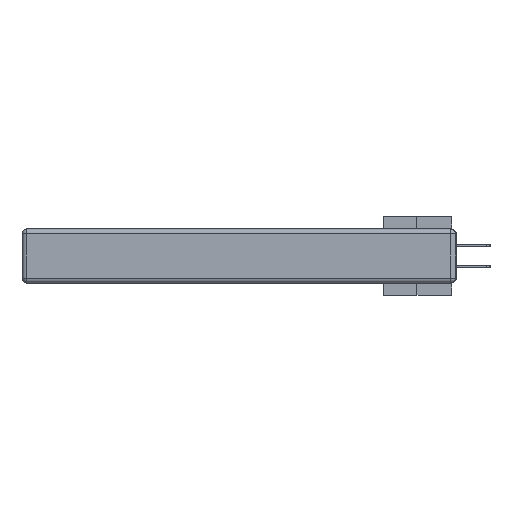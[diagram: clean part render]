
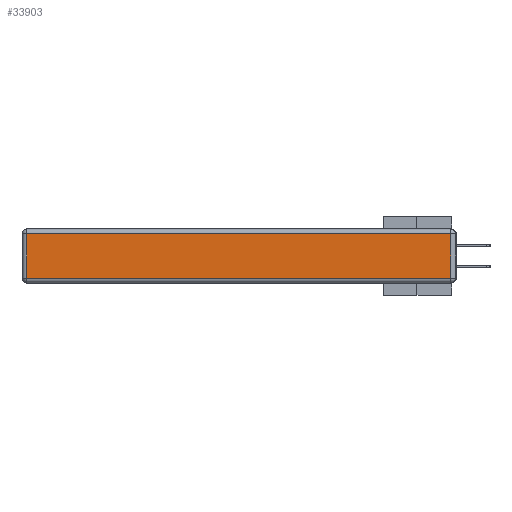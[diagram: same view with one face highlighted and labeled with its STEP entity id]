
A CAD part, left-side view. The second image highlights one B-rep face of the part: STEP entity #33903.
In plain terms, the highlighted planar face has unit normal (-1, 0, 0).
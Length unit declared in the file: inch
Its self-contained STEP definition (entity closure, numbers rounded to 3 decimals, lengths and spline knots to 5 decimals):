
#433 = VERTEX_POINT ( 'NONE', #36442 ) ;
#593 = DIRECTION ( 'NONE',  ( -1., 0., 0. ) ) ;
#1270 = ORIENTED_EDGE ( 'NONE', *, *, #34330, .T. ) ;
#1460 = DIRECTION ( 'NONE',  ( 0., 0., -1. ) ) ;
#1658 = VECTOR ( 'NONE', #24372, 39.37008 ) ;
#2230 = CARTESIAN_POINT ( 'NONE',  ( 0., 2.72, -0.313 ) ) ;
#3919 = ORIENTED_EDGE ( 'NONE', *, *, #25011, .T. ) ;
#5621 = EDGE_CURVE ( 'NONE', #29879, #16397, #23557, .T. ) ;
#6476 = CARTESIAN_POINT ( 'NONE',  ( 0., 2.72, -0.03 ) ) ;
#8736 = LINE ( 'NONE', #32435, #29764 ) ;
#9277 = VERTEX_POINT ( 'NONE', #2230 ) ;
#10388 = DIRECTION ( 'NONE',  ( 0., 0., 1. ) ) ;
#11237 = DIRECTION ( 'NONE',  ( 0., 1., 0. ) ) ;
#11420 = CARTESIAN_POINT ( 'NONE',  ( 0., 0., -0.313 ) ) ;
#13267 = DIRECTION ( 'NONE',  ( 0., 0., 1. ) ) ;
#14525 = VECTOR ( 'NONE', #11237, 39.37008 ) ;
#16397 = VERTEX_POINT ( 'NONE', #6476 ) ;
#17071 = ORIENTED_EDGE ( 'NONE', *, *, #5621, .T. ) ;
#19398 = EDGE_LOOP ( 'NONE', ( #3919, #1270, #17071, #27978 ) ) ;
#19709 = PLANE ( 'NONE',  #41327 ) ;
#19716 = LINE ( 'NONE', #20578, #41203 ) ;
#20578 = CARTESIAN_POINT ( 'NONE',  ( 0., 2.72, -0.343 ) ) ;
#20643 = LINE ( 'NONE', #11420, #1658 ) ;
#22280 = FACE_OUTER_BOUND ( 'NONE', #19398, .T. ) ;
#22483 = EDGE_CURVE ( 'NONE', #16397, #9277, #19716, .T. ) ;
#23557 = LINE ( 'NONE', #33349, #14525 ) ;
#24372 = DIRECTION ( 'NONE',  ( 0., -1., 0. ) ) ;
#25011 = EDGE_CURVE ( 'NONE', #9277, #433, #20643, .T. ) ;
#27978 = ORIENTED_EDGE ( 'NONE', *, *, #22483, .T. ) ;
#29764 = VECTOR ( 'NONE', #13267, 39.37008 ) ;
#29879 = VERTEX_POINT ( 'NONE', #40843 ) ;
#32435 = CARTESIAN_POINT ( 'NONE',  ( 0., 0.03, -0.343 ) ) ;
#33349 = CARTESIAN_POINT ( 'NONE',  ( 0., 2.75, -0.03 ) ) ;
#33903 = ADVANCED_FACE ( 'NONE', ( #22280 ), #19709, .T. ) ;
#34330 = EDGE_CURVE ( 'NONE', #433, #29879, #8736, .T. ) ;
#35718 = CARTESIAN_POINT ( 'NONE',  ( 0., 0., -0.343 ) ) ;
#36442 = CARTESIAN_POINT ( 'NONE',  ( 0., 0.03, -0.313 ) ) ;
#40843 = CARTESIAN_POINT ( 'NONE',  ( 0., 0.03, -0.03 ) ) ;
#41203 = VECTOR ( 'NONE', #1460, 39.37008 ) ;
#41327 = AXIS2_PLACEMENT_3D ( 'NONE', #35718, #593, #10388 ) ;
